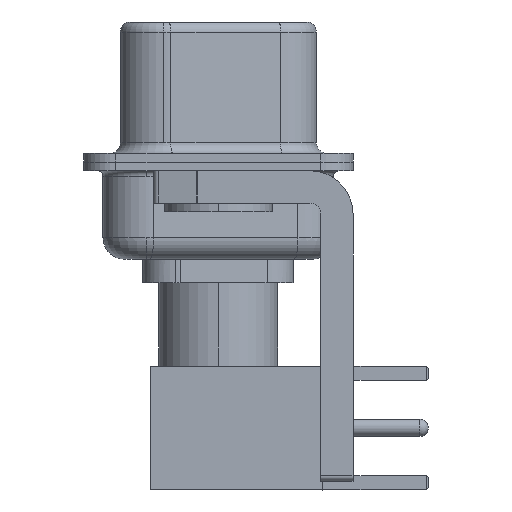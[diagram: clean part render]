
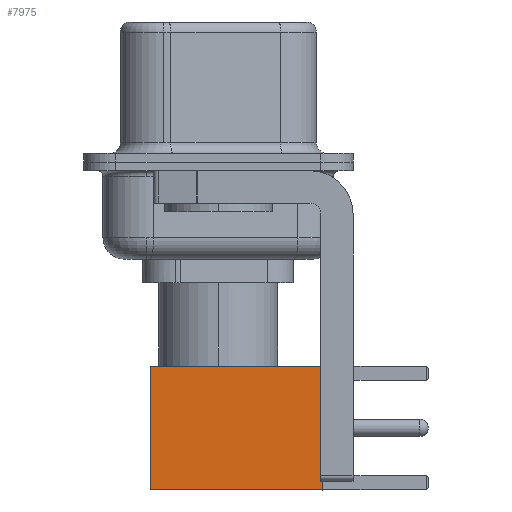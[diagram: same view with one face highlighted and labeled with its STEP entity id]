
A CAD part, left-side view. The second image highlights one B-rep face of the part: STEP entity #7975.
In plain terms, the highlighted face is planar.
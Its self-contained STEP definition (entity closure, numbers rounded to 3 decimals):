
#1337 = DIRECTION ( 'NONE',  ( -1., 0., 0. ) ) ;
#1702 = CARTESIAN_POINT ( 'NONE',  ( 2.875, 2.875, 0. ) ) ;
#2142 = VECTOR ( 'NONE', #14245, 1000. ) ;
#3233 = EDGE_CURVE ( 'NONE', #5774, #16175, #19494, .T. ) ;
#3562 = DIRECTION ( 'NONE',  ( 0., 1., 0. ) ) ;
#5522 = CARTESIAN_POINT ( 'NONE',  ( -2.875, 2.875, 0. ) ) ;
#5774 = VERTEX_POINT ( 'NONE', #13722 ) ;
#6374 = ORIENTED_EDGE ( 'NONE', *, *, #8475, .F. ) ;
#6469 = VECTOR ( 'NONE', #9222, 1000. ) ;
#7295 = PLANE ( 'NONE',  #11796 ) ;
#7975 = ADVANCED_FACE ( 'NONE', ( #17655 ), #7295, .T. ) ;
#8297 = VERTEX_POINT ( 'NONE', #20417 ) ;
#8475 = EDGE_CURVE ( 'NONE', #16777, #16175, #9120, .T. ) ;
#9120 = LINE ( 'NONE', #5522, #2142 ) ;
#9222 = DIRECTION ( 'NONE',  ( 0., 0., -1. ) ) ;
#9911 = DIRECTION ( 'NONE',  ( -1., 0., 0. ) ) ;
#10639 = CARTESIAN_POINT ( 'NONE',  ( 0., 2.875, 0. ) ) ;
#10732 = LINE ( 'NONE', #18072, #6469 ) ;
#11168 = CARTESIAN_POINT ( 'NONE',  ( -2.875, 2.875, 8. ) ) ;
#11221 = VECTOR ( 'NONE', #9911, 1000. ) ;
#11796 = AXIS2_PLACEMENT_3D ( 'NONE', #1702, #3562, #21139 ) ;
#12027 = ORIENTED_EDGE ( 'NONE', *, *, #16090, .F. ) ;
#13285 = LINE ( 'NONE', #22156, #11221 ) ;
#13516 = ORIENTED_EDGE ( 'NONE', *, *, #3233, .T. ) ;
#13722 = CARTESIAN_POINT ( 'NONE',  ( 2.875, 2.875, 0. ) ) ;
#14245 = DIRECTION ( 'NONE',  ( 0., 0., -1. ) ) ;
#14416 = ORIENTED_EDGE ( 'NONE', *, *, #21042, .T. ) ;
#16024 = EDGE_LOOP ( 'NONE', ( #14416, #13516, #6374, #12027 ) ) ;
#16090 = EDGE_CURVE ( 'NONE', #8297, #16777, #13285, .T. ) ;
#16175 = VERTEX_POINT ( 'NONE', #19747 ) ;
#16354 = VECTOR ( 'NONE', #1337, 1000. ) ;
#16777 = VERTEX_POINT ( 'NONE', #11168 ) ;
#17655 = FACE_OUTER_BOUND ( 'NONE', #16024, .T. ) ;
#18072 = CARTESIAN_POINT ( 'NONE',  ( 2.875, 2.875, 0. ) ) ;
#19494 = LINE ( 'NONE', #10639, #16354 ) ;
#19747 = CARTESIAN_POINT ( 'NONE',  ( -2.875, 2.875, 0. ) ) ;
#20417 = CARTESIAN_POINT ( 'NONE',  ( 2.875, 2.875, 8. ) ) ;
#21042 = EDGE_CURVE ( 'NONE', #8297, #5774, #10732, .T. ) ;
#21139 = DIRECTION ( 'NONE',  ( 0., 0., 1. ) ) ;
#22156 = CARTESIAN_POINT ( 'NONE',  ( 0., 2.875, 8. ) ) ;
